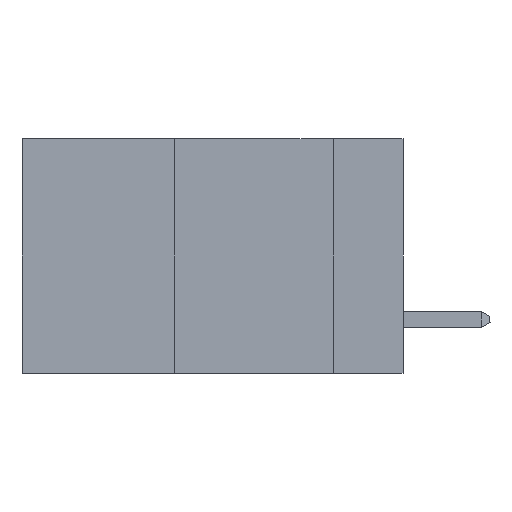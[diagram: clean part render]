
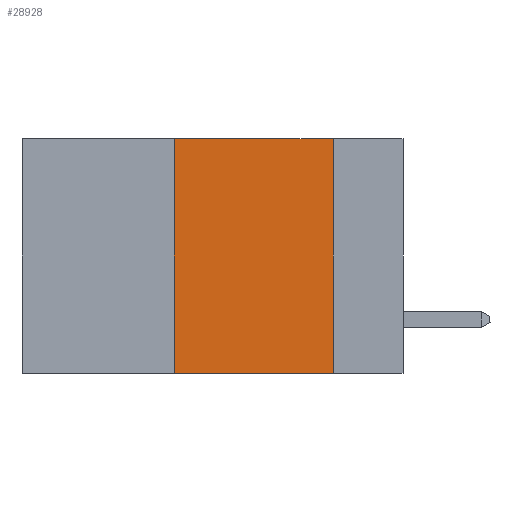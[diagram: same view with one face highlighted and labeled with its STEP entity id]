
A CAD part, left-side view. The second image highlights one B-rep face of the part: STEP entity #28928.
In plain terms, the highlighted planar face has unit normal (-1, 0, 0).
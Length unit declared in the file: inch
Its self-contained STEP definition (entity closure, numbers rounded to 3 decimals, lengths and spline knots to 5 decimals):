
#1871 = LINE ( 'NONE', #6409, #29332 ) ;
#2760 = LINE ( 'NONE', #19764, #27460 ) ;
#2881 = EDGE_CURVE ( 'NONE', #8749, #5905, #2760, .T. ) ;
#3394 = ORIENTED_EDGE ( 'NONE', *, *, #15414, .F. ) ;
#3824 = ORIENTED_EDGE ( 'NONE', *, *, #2881, .T. ) ;
#4086 = EDGE_CURVE ( 'NONE', #8749, #32034, #1871, .T. ) ;
#4247 = DIRECTION ( 'NONE',  ( 0., -1., 0. ) ) ;
#4444 = ORIENTED_EDGE ( 'NONE', *, *, #18494, .F. ) ;
#4800 = CARTESIAN_POINT ( 'NONE',  ( 0., 0.11, 0. ) ) ;
#5416 = LINE ( 'NONE', #16321, #15816 ) ;
#5905 = VERTEX_POINT ( 'NONE', #24750 ) ;
#6409 = CARTESIAN_POINT ( 'NONE',  ( 0., 0.36, 0. ) ) ;
#7798 = CARTESIAN_POINT ( 'NONE',  ( 0., 0.6, 0. ) ) ;
#8749 = VERTEX_POINT ( 'NONE', #31156 ) ;
#8940 = DIRECTION ( 'NONE',  ( 0., -1., 0. ) ) ;
#11556 = LINE ( 'NONE', #28438, #13559 ) ;
#12700 = PLANE ( 'NONE',  #22625 ) ;
#13559 = VECTOR ( 'NONE', #25448, 39.37008 ) ;
#15171 = DIRECTION ( 'NONE',  ( 0., 0., -1. ) ) ;
#15414 = EDGE_CURVE ( 'NONE', #32034, #25837, #5416, .T. ) ;
#15816 = VECTOR ( 'NONE', #8940, 39.37008 ) ;
#16321 = CARTESIAN_POINT ( 'NONE',  ( 0., 0.6, 0. ) ) ;
#18494 = EDGE_CURVE ( 'NONE', #25837, #5905, #11556, .T. ) ;
#19724 = CARTESIAN_POINT ( 'NONE',  ( 0., 0.36, 0. ) ) ;
#19764 = CARTESIAN_POINT ( 'NONE',  ( 0., 0.6, -0.37 ) ) ;
#22625 = AXIS2_PLACEMENT_3D ( 'NONE', #7798, #28186, #15171 ) ;
#24040 = DIRECTION ( 'NONE',  ( 0., 0., 1. ) ) ;
#24588 = ORIENTED_EDGE ( 'NONE', *, *, #4086, .F. ) ;
#24750 = CARTESIAN_POINT ( 'NONE',  ( 0., 0.11, -0.37 ) ) ;
#25448 = DIRECTION ( 'NONE',  ( 0., 0., -1. ) ) ;
#25837 = VERTEX_POINT ( 'NONE', #4800 ) ;
#27460 = VECTOR ( 'NONE', #4247, 39.37008 ) ;
#28186 = DIRECTION ( 'NONE',  ( 1., 0., 0. ) ) ;
#28438 = CARTESIAN_POINT ( 'NONE',  ( 0., 0.11, 0. ) ) ;
#28928 = ADVANCED_FACE ( 'NONE', ( #29135 ), #12700, .F. ) ;
#29135 = FACE_OUTER_BOUND ( 'NONE', #29584, .T. ) ;
#29332 = VECTOR ( 'NONE', #24040, 39.37008 ) ;
#29584 = EDGE_LOOP ( 'NONE', ( #4444, #3394, #24588, #3824 ) ) ;
#31156 = CARTESIAN_POINT ( 'NONE',  ( 0., 0.36, -0.37 ) ) ;
#32034 = VERTEX_POINT ( 'NONE', #19724 ) ;
